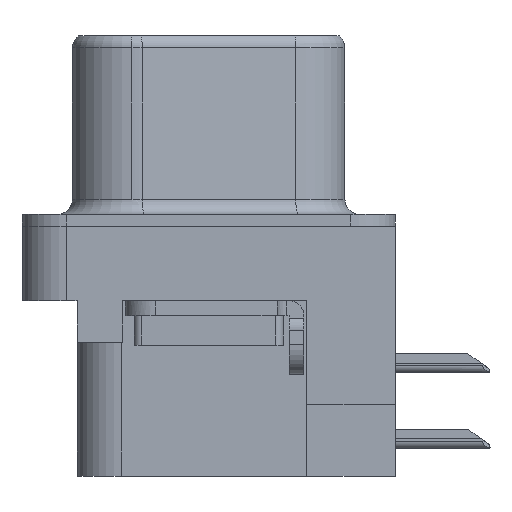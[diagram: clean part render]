
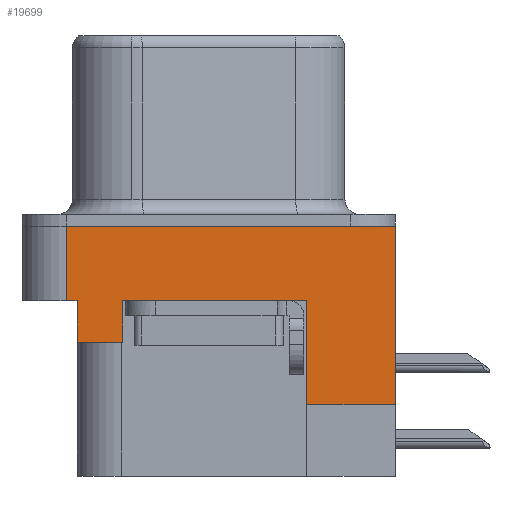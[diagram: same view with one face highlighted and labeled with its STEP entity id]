
A CAD part, left-side view. The second image highlights one B-rep face of the part: STEP entity #19699.
In plain terms, the highlighted planar face has unit normal (-1, 0, 0).
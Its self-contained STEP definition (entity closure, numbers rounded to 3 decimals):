
#119 = CARTESIAN_POINT ( 'NONE',  ( -3., 4.775, -2.5 ) ) ;
#301 = CARTESIAN_POINT ( 'NONE',  ( -3., 4.425, -3.9 ) ) ;
#403 = LINE ( 'NONE', #15315, #508 ) ;
#482 = DIRECTION ( 'NONE',  ( 0., 0., 1. ) ) ;
#489 = LINE ( 'NONE', #559, #554 ) ;
#508 = VECTOR ( 'NONE', #14793, 1000. ) ;
#554 = VECTOR ( 'NONE', #482, 1000. ) ;
#559 = CARTESIAN_POINT ( 'NONE',  ( -3., -6.275, -2.5 ) ) ;
#643 = VERTEX_POINT ( 'NONE', #9783 ) ;
#773 = VERTEX_POINT ( 'NONE', #9641 ) ;
#1246 = DIRECTION ( 'NONE',  ( 0., 0., 1. ) ) ;
#1574 = EDGE_CURVE ( 'NONE', #16218, #20775, #5337, .T. ) ;
#1640 = VECTOR ( 'NONE', #2037, 1000. ) ;
#1679 = EDGE_CURVE ( 'NONE', #8487, #10968, #4905, .T. ) ;
#1702 = LINE ( 'NONE', #12647, #1717 ) ;
#1717 = VECTOR ( 'NONE', #9952, 1000. ) ;
#1781 = LINE ( 'NONE', #14157, #1640 ) ;
#1845 = LINE ( 'NONE', #6344, #1866 ) ;
#1866 = VECTOR ( 'NONE', #4630, 1000. ) ;
#2037 = DIRECTION ( 'NONE',  ( 0., -1., 0. ) ) ;
#2118 = LINE ( 'NONE', #12982, #2396 ) ;
#2180 = EDGE_CURVE ( 'NONE', #643, #7278, #2118, .T. ) ;
#2254 = EDGE_CURVE ( 'NONE', #20775, #10968, #1845, .T. ) ;
#2278 = EDGE_CURVE ( 'NONE', #8487, #17723, #1702, .T. ) ;
#2279 = EDGE_CURVE ( 'NONE', #17723, #773, #1781, .T. ) ;
#2396 = VECTOR ( 'NONE', #1246, 1000. ) ;
#2489 = EDGE_CURVE ( 'NONE', #11499, #773, #489, .T. ) ;
#2523 = EDGE_CURVE ( 'NONE', #11499, #643, #403, .T. ) ;
#2666 = ORIENTED_EDGE ( 'NONE', *, *, #2489, .T. ) ;
#3180 = EDGE_CURVE ( 'NONE', #16218, #3820, #18646, .T. ) ;
#3382 = CARTESIAN_POINT ( 'NONE',  ( -3., -3.295, -2.5 ) ) ;
#3385 = CARTESIAN_POINT ( 'NONE',  ( -3., -6.275, -2.5 ) ) ;
#3691 = ORIENTED_EDGE ( 'NONE', *, *, #3180, .T. ) ;
#3820 = VERTEX_POINT ( 'NONE', #12817 ) ;
#4228 = CARTESIAN_POINT ( 'NONE',  ( -3., 4.775, 0. ) ) ;
#4519 = EDGE_CURVE ( 'NONE', #3820, #7278, #12459, .T. ) ;
#4630 = DIRECTION ( 'NONE',  ( 0., 0., 1. ) ) ;
#4709 = DIRECTION ( 'NONE',  ( 0., -1., 0. ) ) ;
#4828 = VECTOR ( 'NONE', #4709, 1000. ) ;
#4905 = LINE ( 'NONE', #6615, #4828 ) ;
#5276 = VECTOR ( 'NONE', #18140, 1000. ) ;
#5337 = LINE ( 'NONE', #301, #5276 ) ;
#5558 = ORIENTED_EDGE ( 'NONE', *, *, #2278, .F. ) ;
#6344 = CARTESIAN_POINT ( 'NONE',  ( -3., 4.425, -3.9 ) ) ;
#6416 = AXIS2_PLACEMENT_3D ( 'NONE', #17907, #21245, #16247 ) ;
#6615 = CARTESIAN_POINT ( 'NONE',  ( -3., -6.275, -2.5 ) ) ;
#7278 = VERTEX_POINT ( 'NONE', #3382 ) ;
#7309 = CARTESIAN_POINT ( 'NONE',  ( -3., 2.895, -3.9 ) ) ;
#7454 = ORIENTED_EDGE ( 'NONE', *, *, #1679, .T. ) ;
#8388 = DIRECTION ( 'NONE',  ( 0., 0., 1. ) ) ;
#8487 = VERTEX_POINT ( 'NONE', #119 ) ;
#9641 = CARTESIAN_POINT ( 'NONE',  ( -3., -6.275, 0. ) ) ;
#9783 = CARTESIAN_POINT ( 'NONE',  ( -3., -3.295, -6. ) ) ;
#9952 = DIRECTION ( 'NONE',  ( 0., 0., 1. ) ) ;
#10180 = FACE_OUTER_BOUND ( 'NONE', #16479, .T. ) ;
#10968 = VERTEX_POINT ( 'NONE', #11643 ) ;
#11499 = VERTEX_POINT ( 'NONE', #12939 ) ;
#11643 = CARTESIAN_POINT ( 'NONE',  ( -3., 4.425, -2.5 ) ) ;
#11827 = ORIENTED_EDGE ( 'NONE', *, *, #2523, .F. ) ;
#12118 = ORIENTED_EDGE ( 'NONE', *, *, #1574, .F. ) ;
#12411 = VECTOR ( 'NONE', #20191, 1000. ) ;
#12459 = LINE ( 'NONE', #3385, #12411 ) ;
#12647 = CARTESIAN_POINT ( 'NONE',  ( -3., 4.775, -2.5 ) ) ;
#12752 = PLANE ( 'NONE',  #6416 ) ;
#12817 = CARTESIAN_POINT ( 'NONE',  ( -3., 2.895, -2.5 ) ) ;
#12939 = CARTESIAN_POINT ( 'NONE',  ( -3., -6.275, -6. ) ) ;
#12982 = CARTESIAN_POINT ( 'NONE',  ( -3., -3.295, -8.4 ) ) ;
#14157 = CARTESIAN_POINT ( 'NONE',  ( -3., -6.275, 0. ) ) ;
#14793 = DIRECTION ( 'NONE',  ( 0., 1., 0. ) ) ;
#15315 = CARTESIAN_POINT ( 'NONE',  ( -3., -6.495, -6. ) ) ;
#16218 = VERTEX_POINT ( 'NONE', #7309 ) ;
#16247 = DIRECTION ( 'NONE',  ( 0., 0., 1. ) ) ;
#16479 = EDGE_LOOP ( 'NONE', ( #11827, #2666, #21025, #5558, #7454, #21416, #12118, #3691, #19826, #20736 ) ) ;
#17723 = VERTEX_POINT ( 'NONE', #4228 ) ;
#17907 = CARTESIAN_POINT ( 'NONE',  ( -3., -6.275, -2.5 ) ) ;
#18140 = DIRECTION ( 'NONE',  ( 0., 1., 0. ) ) ;
#18646 = LINE ( 'NONE', #19748, #18742 ) ;
#18742 = VECTOR ( 'NONE', #8388, 1000. ) ;
#19052 = CARTESIAN_POINT ( 'NONE',  ( -3., 4.425, -3.9 ) ) ;
#19699 = ADVANCED_FACE ( 'NONE', ( #10180 ), #12752, .T. ) ;
#19748 = CARTESIAN_POINT ( 'NONE',  ( -3., 2.895, -3.9 ) ) ;
#19826 = ORIENTED_EDGE ( 'NONE', *, *, #4519, .T. ) ;
#20191 = DIRECTION ( 'NONE',  ( 0., -1., 0. ) ) ;
#20736 = ORIENTED_EDGE ( 'NONE', *, *, #2180, .F. ) ;
#20775 = VERTEX_POINT ( 'NONE', #19052 ) ;
#21025 = ORIENTED_EDGE ( 'NONE', *, *, #2279, .F. ) ;
#21245 = DIRECTION ( 'NONE',  ( -1., 0., 0. ) ) ;
#21416 = ORIENTED_EDGE ( 'NONE', *, *, #2254, .F. ) ;
